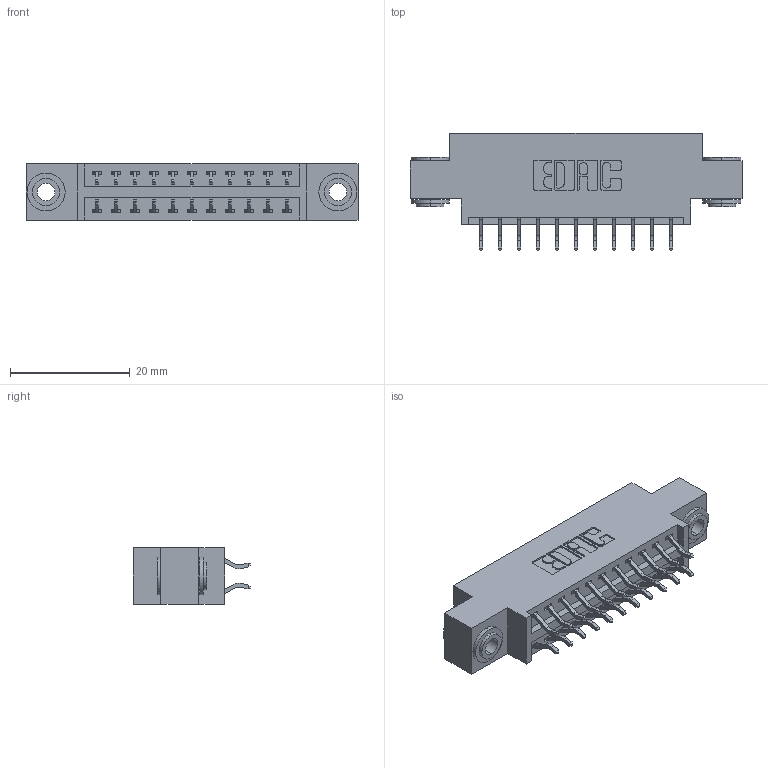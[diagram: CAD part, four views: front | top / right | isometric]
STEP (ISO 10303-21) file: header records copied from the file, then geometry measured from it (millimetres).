
FILE_DESCRIPTION (( 'STEP AP203' ), '1' );
FILE_NAME ('396-022-556-803.STEP', '2019-11-01T18:33:46', ( '' ), ( '' ), 'SwSTEP 2.0', 'SolidWorks 2016', '' );
FILE_SCHEMA (( 'CONFIG_CONTROL_DESIGN' ));
Length unit declared in the file: inch
Products named in the file (4): 346 Part_0.170 Offset - 0.156 Dia-TH; 345-292-001_556 Tail; 345-250-002_345-250-002-102; 396-022-556-803
Assembly tree (25 placements, depth 2):
  396-022-556-803
    346 Part_0.170 Offset - 0.156 Dia-TH
    345-292-001_556 Tail  x22
    345-250-002_345-250-002-102  x2
Bounding box: 55.5 x 19.57 x 9.4 mm (x, y, z)
Volume: 5035 mm3; surface area: 6807 mm2
Topology: 25 solids, 25 shells, 1440 faces, 4223 edges, 2782 vertices
Faces by surface type: plane 948, cylinder 484, cone 8
Entity records: 12354 total; most frequent: CARTESIAN_POINT 2071, ORIENTED_EDGE 1986, DIRECTION 1895, EDGE_CURVE 993, LINE 785, VECTOR 785, VERTEX_POINT 658, AXIS2_PLACEMENT_3D 555
